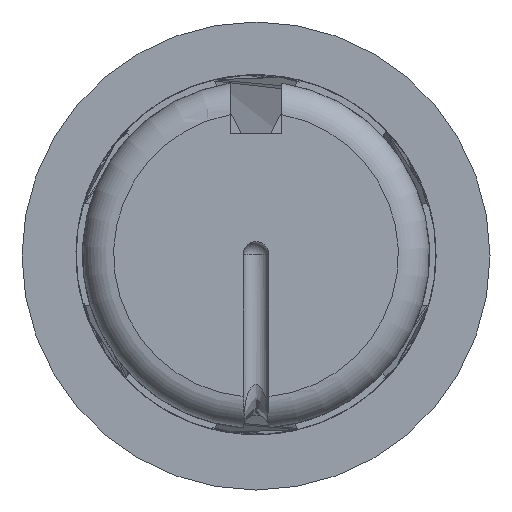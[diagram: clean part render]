
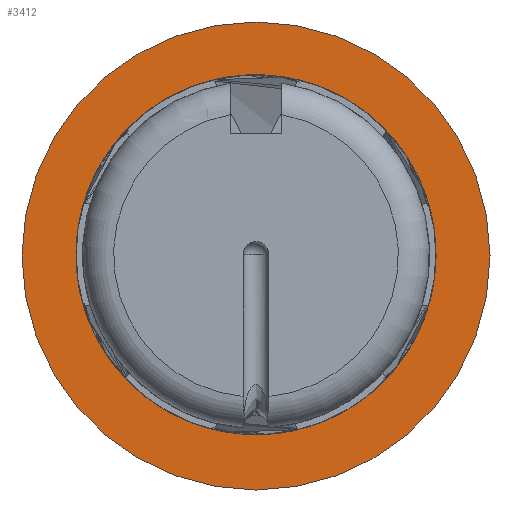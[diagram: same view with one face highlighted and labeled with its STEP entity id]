
A CAD part, front view. The second image highlights one B-rep face of the part: STEP entity #3412.
In plain terms, the highlighted planar face has unit normal (0, -1, 0).
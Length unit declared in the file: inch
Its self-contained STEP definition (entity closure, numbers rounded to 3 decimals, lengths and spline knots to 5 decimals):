
#44=FACE_BOUND('',#527,.T.);
#59=PLANE('',#3584);
#106=CIRCLE('',#3513,0.17362);
#107=CIRCLE('',#3514,0.17362);
#125=CIRCLE('',#3552,0.22566);
#338=FACE_OUTER_BOUND('',#526,.T.);
#526=EDGE_LOOP('',(#2999));
#527=EDGE_LOOP('',(#3000,#3001));
#1297=VERTEX_POINT('',#6319);
#1298=VERTEX_POINT('',#6320);
#1418=VERTEX_POINT('',#7811);
#1737=EDGE_CURVE('',#1297,#1298,#106,.T.);
#1739=EDGE_CURVE('',#1298,#1297,#107,.T.);
#1914=EDGE_CURVE('',#1418,#1418,#125,.T.);
#2999=ORIENTED_EDGE('',*,*,#1914,.F.);
#3000=ORIENTED_EDGE('',*,*,#1737,.F.);
#3001=ORIENTED_EDGE('',*,*,#1739,.F.);
#3412=ADVANCED_FACE('',(#338,#44),#59,.T.);
#3513=AXIS2_PLACEMENT_3D('',#6321,#3749,#3750);
#3514=AXIS2_PLACEMENT_3D('',#6323,#3752,#3753);
#3552=AXIS2_PLACEMENT_3D('',#7813,#3837,#3838);
#3584=AXIS2_PLACEMENT_3D('',#8821,#3906,#3907);
#3749=DIRECTION('center_axis',(0.,-1.,0.));
#3750=DIRECTION('ref_axis',(-1.,0.,0.));
#3752=DIRECTION('center_axis',(0.,-1.,0.));
#3753=DIRECTION('ref_axis',(-1.,0.,0.));
#3837=DIRECTION('center_axis',(0.,1.,0.));
#3838=DIRECTION('ref_axis',(1.,0.,0.));
#3906=DIRECTION('center_axis',(0.,-1.,0.));
#3907=DIRECTION('ref_axis',(0.,0.,-1.));
#6319=CARTESIAN_POINT('',(0.17362,5.28877,0.));
#6320=CARTESIAN_POINT('',(0.17352,5.28877,-0.0059));
#6321=CARTESIAN_POINT('Origin',(0.,5.28877,0.));
#6323=CARTESIAN_POINT('Origin',(0.,5.28877,0.));
#7811=CARTESIAN_POINT('',(0.22566,5.28877,-0.00126));
#7813=CARTESIAN_POINT('Origin',(0.,5.28877,-0.00126));
#8821=CARTESIAN_POINT('Origin',(0.,5.28877,0.2244));
